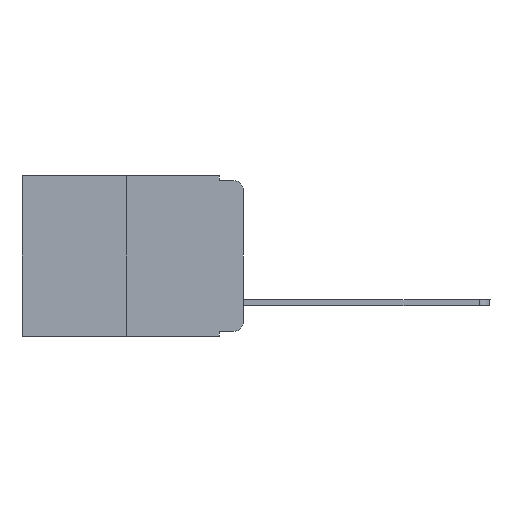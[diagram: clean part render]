
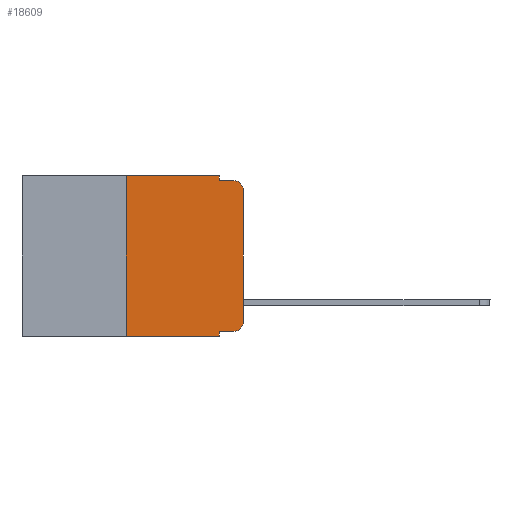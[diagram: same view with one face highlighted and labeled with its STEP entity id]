
A CAD part, left-side view. The second image highlights one B-rep face of the part: STEP entity #18609.
In plain terms, the highlighted planar face has unit normal (-1, 0, 0).
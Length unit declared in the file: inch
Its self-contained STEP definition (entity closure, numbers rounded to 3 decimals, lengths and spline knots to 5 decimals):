
#512 = CARTESIAN_POINT ( 'NONE',  ( 0., 0.02, -0.313 ) ) ;
#546 = VERTEX_POINT ( 'NONE', #11689 ) ;
#1648 = ORIENTED_EDGE ( 'NONE', *, *, #2774, .T. ) ;
#1693 = LINE ( 'NONE', #12951, #7104 ) ;
#2149 = VERTEX_POINT ( 'NONE', #7753 ) ;
#2178 = DIRECTION ( 'NONE',  ( 0., 0., -1. ) ) ;
#2204 = EDGE_CURVE ( 'NONE', #2149, #546, #20242, .T. ) ;
#2354 = VERTEX_POINT ( 'NONE', #13635 ) ;
#2507 = VECTOR ( 'NONE', #10008, 39.37008 ) ;
#2519 = DIRECTION ( 'NONE',  ( 0., 0., 1. ) ) ;
#2573 = DIRECTION ( 'NONE',  ( 0., 0., -1. ) ) ;
#2774 = EDGE_CURVE ( 'NONE', #15811, #10409, #16543, .T. ) ;
#3323 = VECTOR ( 'NONE', #7837, 39.37008 ) ;
#3557 = EDGE_LOOP ( 'NONE', ( #4463, #1648, #12433, #7065, #19663, #6124, #5986, #3633, #14119, #19589 ) ) ;
#3568 = DIRECTION ( 'NONE',  ( 0., -1., 0. ) ) ;
#3633 = ORIENTED_EDGE ( 'NONE', *, *, #13066, .F. ) ;
#3745 = EDGE_CURVE ( 'NONE', #19624, #2149, #13199, .T. ) ;
#3922 = CARTESIAN_POINT ( 'NONE',  ( 0., 0.473, 0. ) ) ;
#4463 = ORIENTED_EDGE ( 'NONE', *, *, #14542, .T. ) ;
#5497 = EDGE_CURVE ( 'NONE', #17481, #16737, #21078, .T. ) ;
#5986 = ORIENTED_EDGE ( 'NONE', *, *, #17105, .T. ) ;
#6124 = ORIENTED_EDGE ( 'NONE', *, *, #13187, .F. ) ;
#7065 = ORIENTED_EDGE ( 'NONE', *, *, #2204, .F. ) ;
#7104 = VECTOR ( 'NONE', #3568, 39.37008 ) ;
#7374 = DIRECTION ( 'NONE',  ( 1., 0., 0. ) ) ;
#7391 = LINE ( 'NONE', #12526, #8673 ) ;
#7753 = CARTESIAN_POINT ( 'NONE',  ( 0., 0.051, 0. ) ) ;
#7837 = DIRECTION ( 'NONE',  ( 0., 0., -1. ) ) ;
#7938 = EDGE_CURVE ( 'NONE', #2354, #17481, #1693, .T. ) ;
#8093 = VERTEX_POINT ( 'NONE', #8394 ) ;
#8111 = AXIS2_PLACEMENT_3D ( 'NONE', #512, #12079, #2573 ) ;
#8394 = CARTESIAN_POINT ( 'NONE',  ( 0., 0.051, -0.343 ) ) ;
#8515 = CARTESIAN_POINT ( 'NONE',  ( 0., 0.02, -0.01 ) ) ;
#8673 = VECTOR ( 'NONE', #2519, 39.37008 ) ;
#8911 = DIRECTION ( 'NONE',  ( 0., -1., 0. ) ) ;
#9193 = VECTOR ( 'NONE', #16262, 39.37008 ) ;
#9396 = CARTESIAN_POINT ( 'NONE',  ( 0., 0., -0.03 ) ) ;
#9442 = CARTESIAN_POINT ( 'NONE',  ( 0., 0.051, 0. ) ) ;
#9547 = AXIS2_PLACEMENT_3D ( 'NONE', #3922, #7374, #18869 ) ;
#9566 = VERTEX_POINT ( 'NONE', #10189 ) ;
#9934 = CARTESIAN_POINT ( 'NONE',  ( 0., 0.051, 0. ) ) ;
#10008 = DIRECTION ( 'NONE',  ( 0., 0., -1. ) ) ;
#10126 = LINE ( 'NONE', #20525, #12923 ) ;
#10189 = CARTESIAN_POINT ( 'NONE',  ( 0., 0.25, -0.343 ) ) ;
#10409 = VERTEX_POINT ( 'NONE', #8515 ) ;
#10916 = EDGE_CURVE ( 'NONE', #546, #10409, #10126, .T. ) ;
#11654 = DIRECTION ( 'NONE',  ( 0., 0., 1. ) ) ;
#11689 = CARTESIAN_POINT ( 'NONE',  ( 0., 0.051, -0.01 ) ) ;
#12079 = DIRECTION ( 'NONE',  ( -1., 0., 0. ) ) ;
#12274 = CARTESIAN_POINT ( 'NONE',  ( 0., 0.02, -0.333 ) ) ;
#12433 = ORIENTED_EDGE ( 'NONE', *, *, #10916, .F. ) ;
#12526 = CARTESIAN_POINT ( 'NONE',  ( 0., 0., 0. ) ) ;
#12607 = LINE ( 'NONE', #9442, #3323 ) ;
#12923 = VECTOR ( 'NONE', #8911, 39.37008 ) ;
#12951 = CARTESIAN_POINT ( 'NONE',  ( 0., 0.051, -0.333 ) ) ;
#13066 = EDGE_CURVE ( 'NONE', #2354, #8093, #12607, .T. ) ;
#13078 = CARTESIAN_POINT ( 'NONE',  ( 0., 0.25, 0. ) ) ;
#13148 = CARTESIAN_POINT ( 'NONE',  ( 0., 0., -0.313 ) ) ;
#13187 = EDGE_CURVE ( 'NONE', #9566, #19624, #14382, .T. ) ;
#13199 = LINE ( 'NONE', #18535, #19132 ) ;
#13635 = CARTESIAN_POINT ( 'NONE',  ( 0., 0.051, -0.333 ) ) ;
#14119 = ORIENTED_EDGE ( 'NONE', *, *, #7938, .T. ) ;
#14174 = CARTESIAN_POINT ( 'NONE',  ( 0., 0.473, -0.343 ) ) ;
#14382 = LINE ( 'NONE', #13078, #17202 ) ;
#14542 = EDGE_CURVE ( 'NONE', #16737, #15811, #7391, .T. ) ;
#15811 = VERTEX_POINT ( 'NONE', #9396 ) ;
#16262 = DIRECTION ( 'NONE',  ( 0., -1., 0. ) ) ;
#16543 = CIRCLE ( 'NONE', #18807, 0.02 ) ;
#16737 = VERTEX_POINT ( 'NONE', #13148 ) ;
#16948 = CARTESIAN_POINT ( 'NONE',  ( 0., 0.02, -0.03 ) ) ;
#17021 = DIRECTION ( 'NONE',  ( -1., 0., 0. ) ) ;
#17078 = DIRECTION ( 'NONE',  ( 0., -1., 0. ) ) ;
#17105 = EDGE_CURVE ( 'NONE', #9566, #8093, #19988, .T. ) ;
#17198 = PLANE ( 'NONE',  #9547 ) ;
#17202 = VECTOR ( 'NONE', #11654, 39.37008 ) ;
#17481 = VERTEX_POINT ( 'NONE', #12274 ) ;
#17888 = CARTESIAN_POINT ( 'NONE',  ( 0., 0.25, 0. ) ) ;
#18535 = CARTESIAN_POINT ( 'NONE',  ( 0., 0.473, 0. ) ) ;
#18609 = ADVANCED_FACE ( 'NONE', ( #20703 ), #17198, .F. ) ;
#18807 = AXIS2_PLACEMENT_3D ( 'NONE', #16948, #17021, #2178 ) ;
#18869 = DIRECTION ( 'NONE',  ( 0., 0., -1. ) ) ;
#19132 = VECTOR ( 'NONE', #17078, 39.37008 ) ;
#19589 = ORIENTED_EDGE ( 'NONE', *, *, #5497, .T. ) ;
#19624 = VERTEX_POINT ( 'NONE', #17888 ) ;
#19663 = ORIENTED_EDGE ( 'NONE', *, *, #3745, .F. ) ;
#19988 = LINE ( 'NONE', #14174, #9193 ) ;
#20242 = LINE ( 'NONE', #9934, #2507 ) ;
#20525 = CARTESIAN_POINT ( 'NONE',  ( 0., 0.051, -0.01 ) ) ;
#20703 = FACE_OUTER_BOUND ( 'NONE', #3557, .T. ) ;
#21078 = CIRCLE ( 'NONE', #8111, 0.02 ) ;
